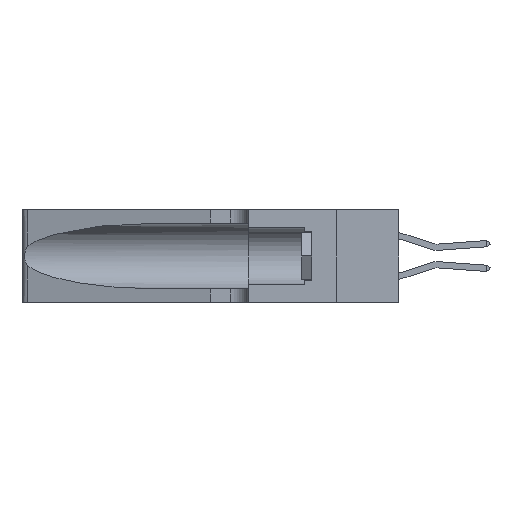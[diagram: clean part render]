
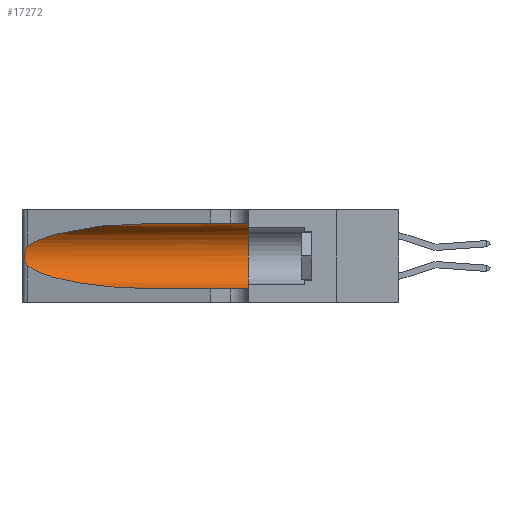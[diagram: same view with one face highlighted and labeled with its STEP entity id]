
A CAD part, left-side view. The second image highlights one B-rep face of the part: STEP entity #17272.
In plain terms, the highlighted cylindrical face has radius 3.308 mm (diameter 6.617 mm), a partial arc.
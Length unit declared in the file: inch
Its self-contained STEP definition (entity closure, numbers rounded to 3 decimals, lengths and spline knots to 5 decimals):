
#829 =( BOUNDED_CURVE ( )  B_SPLINE_CURVE ( 3, ( #10081, #12840, #9947, #15980 ),
 .UNSPECIFIED., .F., .T. ) 
 B_SPLINE_CURVE_WITH_KNOTS ( ( 4, 4 ),
 ( 3.44316, 4.71239 ),
 .UNSPECIFIED. ) 
 CURVE ( )  GEOMETRIC_REPRESENTATION_ITEM ( )  RATIONAL_B_SPLINE_CURVE ( ( 1., 0.87, 0.87, 1. ) ) 
 REPRESENTATION_ITEM ( '' )  );
#1014 = VERTEX_POINT ( 'NONE', #19405 ) ;
#2163 = CARTESIAN_POINT ( 'NONE',  ( 0.2373, 1.15595, 0.28018 ) ) ;
#2674 = ORIENTED_EDGE ( 'NONE', *, *, #24383, .T. ) ;
#4989 = ORIENTED_EDGE ( 'NONE', *, *, #6328, .F. ) ;
#6016 = CARTESIAN_POINT ( 'NONE',  ( 0.1305, 0.35, 0.31525 ) ) ;
#6204 = CIRCLE ( 'NONE', #17899, 0.13025 ) ;
#6328 = EDGE_CURVE ( 'NONE', #36792, #34780, #14290, .T. ) ;
#6663 = CARTESIAN_POINT ( 'NONE',  ( 0.1305, 0.35, 0.185 ) ) ;
#7896 = B_SPLINE_CURVE_WITH_KNOTS ( 'NONE', 3,
 ( #32819, #20393, #15038, #33548, #27515, #21033, #18109, #21283, #24306, #12653, #22045, #13056, #25220, #15530 ),
 .UNSPECIFIED., .F., .F.,
 ( 4, 2, 2, 2, 2, 2, 4 ),
 ( 0., 0.00027, 0.00053, 0.00107, 0.0016, 0.00187, 0.00214 ),
 .UNSPECIFIED. ) ;
#8151 = DIRECTION ( 'NONE',  ( 0., -1., 0. ) ) ;
#8937 = CARTESIAN_POINT ( 'NONE',  ( 0.1305, 1.61858, 0.31525 ) ) ;
#9266 = FACE_OUTER_BOUND ( 'NONE', #36119, .T. ) ;
#9585 = AXIS2_PLACEMENT_3D ( 'NONE', #20420, #8151, #14175 ) ;
#9678 = DIRECTION ( 'NONE',  ( 0., 0., 1. ) ) ;
#9795 = DIRECTION ( 'NONE',  ( 0., -1., 0. ) ) ;
#9947 = CARTESIAN_POINT ( 'NONE',  ( 0.18966, 0.96281, 0.05475 ) ) ;
#10081 = CARTESIAN_POINT ( 'NONE',  ( 0.25487, 1.22718, 0.14631 ) ) ;
#10388 = VERTEX_POINT ( 'NONE', #31642 ) ;
#10955 = DIRECTION ( 'NONE',  ( 0., -1., 0. ) ) ;
#11257 = CARTESIAN_POINT ( 'NONE',  ( 0.25487, 1.22718, 0.22369 ) ) ;
#11533 = EDGE_CURVE ( 'NONE', #1014, #38511, #829, .T. ) ;
#12653 = CARTESIAN_POINT ( 'NONE',  ( 0.25856, 1.23593, 0.16098 ) ) ;
#12840 = CARTESIAN_POINT ( 'NONE',  ( 0.2373, 1.15595, 0.08982 ) ) ;
#13056 = CARTESIAN_POINT ( 'NONE',  ( 0.25639, 1.23186, 0.15144 ) ) ;
#13790 = EDGE_CURVE ( 'NONE', #10388, #1014, #7896, .T. ) ;
#14175 = DIRECTION ( 'NONE',  ( 0., 0., -1. ) ) ;
#14290 = LINE ( 'NONE', #8937, #16150 ) ;
#15038 = CARTESIAN_POINT ( 'NONE',  ( 0.25639, 1.23184, 0.21858 ) ) ;
#15409 = CARTESIAN_POINT ( 'NONE',  ( 0.1305, 0.35, 0.05475 ) ) ;
#15530 = CARTESIAN_POINT ( 'NONE',  ( 0.25487, 1.22718, 0.14631 ) ) ;
#15980 = CARTESIAN_POINT ( 'NONE',  ( 0.1305, 0.72297, 0.05475 ) ) ;
#16150 = VECTOR ( 'NONE', #9795, 39.37008 ) ;
#16763 = CARTESIAN_POINT ( 'NONE',  ( 0.18966, 0.96281, 0.31525 ) ) ;
#17272 = ADVANCED_FACE ( 'NONE', ( #9266 ), #26846, .F. ) ;
#17899 = AXIS2_PLACEMENT_3D ( 'NONE', #6663, #27813, #9678 ) ;
#18109 = CARTESIAN_POINT ( 'NONE',  ( 0.26075, 1.23896, 0.19203 ) ) ;
#19405 = CARTESIAN_POINT ( 'NONE',  ( 0.25487, 1.22718, 0.14631 ) ) ;
#19668 = ORIENTED_EDGE ( 'NONE', *, *, #31634, .T. ) ;
#20393 = CARTESIAN_POINT ( 'NONE',  ( 0.25555, 1.22994, 0.2215 ) ) ;
#20420 = CARTESIAN_POINT ( 'NONE',  ( 0.1305, 1.61858, 0.185 ) ) ;
#21033 = CARTESIAN_POINT ( 'NONE',  ( 0.26018, 1.23835, 0.19895 ) ) ;
#21283 = CARTESIAN_POINT ( 'NONE',  ( 0.26075, 1.23896, 0.178 ) ) ;
#22045 = CARTESIAN_POINT ( 'NONE',  ( 0.25789, 1.23486, 0.15765 ) ) ;
#24306 = CARTESIAN_POINT ( 'NONE',  ( 0.26017, 1.23833, 0.17102 ) ) ;
#24383 = EDGE_CURVE ( 'NONE', #38511, #27417, #35071, .T. ) ;
#25200 = EDGE_CURVE ( 'NONE', #34780, #27417, #6204, .T. ) ;
#25220 = CARTESIAN_POINT ( 'NONE',  ( 0.25555, 1.22993, 0.14849 ) ) ;
#26846 = CYLINDRICAL_SURFACE ( 'NONE', #9585, 0.13025 ) ;
#26853 = CARTESIAN_POINT ( 'NONE',  ( 0.1305, 0.72297, 0.05475 ) ) ;
#27417 = VERTEX_POINT ( 'NONE', #15409 ) ;
#27515 = CARTESIAN_POINT ( 'NONE',  ( 0.25854, 1.2359, 0.20912 ) ) ;
#27644 = CARTESIAN_POINT ( 'NONE',  ( 0.1305, 0.72297, 0.31525 ) ) ;
#27813 = DIRECTION ( 'NONE',  ( 0., 1., 0. ) ) ;
#27993 = VECTOR ( 'NONE', #10955, 39.37008 ) ;
#31488 = ORIENTED_EDGE ( 'NONE', *, *, #11533, .T. ) ;
#31634 = EDGE_CURVE ( 'NONE', #36792, #10388, #34752, .T. ) ;
#31642 = CARTESIAN_POINT ( 'NONE',  ( 0.25487, 1.22718, 0.22369 ) ) ;
#31876 = CARTESIAN_POINT ( 'NONE',  ( 0.1305, 0.72297, 0.31525 ) ) ;
#32387 = CARTESIAN_POINT ( 'NONE',  ( 0.1305, 1.61858, 0.05475 ) ) ;
#32819 = CARTESIAN_POINT ( 'NONE',  ( 0.25487, 1.22718, 0.22369 ) ) ;
#33548 = CARTESIAN_POINT ( 'NONE',  ( 0.25787, 1.23484, 0.2124 ) ) ;
#34246 = ORIENTED_EDGE ( 'NONE', *, *, #13790, .T. ) ;
#34529 = ORIENTED_EDGE ( 'NONE', *, *, #25200, .F. ) ;
#34752 =( BOUNDED_CURVE ( )  B_SPLINE_CURVE ( 3, ( #31876, #16763, #2163, #11257 ),
 .UNSPECIFIED., .F., .F. ) 
 B_SPLINE_CURVE_WITH_KNOTS ( ( 4, 4 ),
 ( 1.5708, 2.84003 ),
 .UNSPECIFIED. ) 
 CURVE ( )  GEOMETRIC_REPRESENTATION_ITEM ( )  RATIONAL_B_SPLINE_CURVE ( ( 1., 0.87, 0.87, 1. ) ) 
 REPRESENTATION_ITEM ( '' )  );
#34780 = VERTEX_POINT ( 'NONE', #6016 ) ;
#35071 = LINE ( 'NONE', #32387, #27993 ) ;
#36119 = EDGE_LOOP ( 'NONE', ( #19668, #34246, #31488, #2674, #34529, #4989 ) ) ;
#36792 = VERTEX_POINT ( 'NONE', #27644 ) ;
#38511 = VERTEX_POINT ( 'NONE', #26853 ) ;
